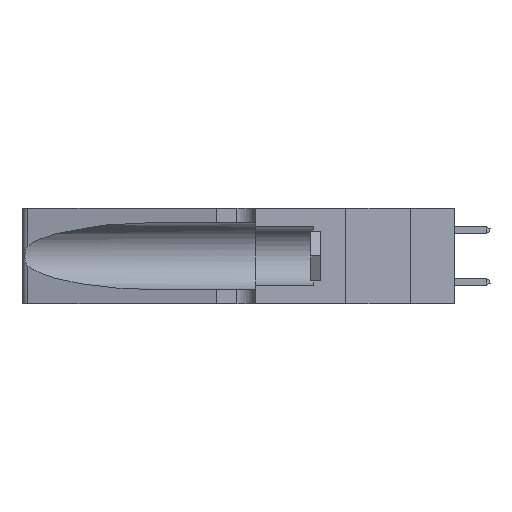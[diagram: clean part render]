
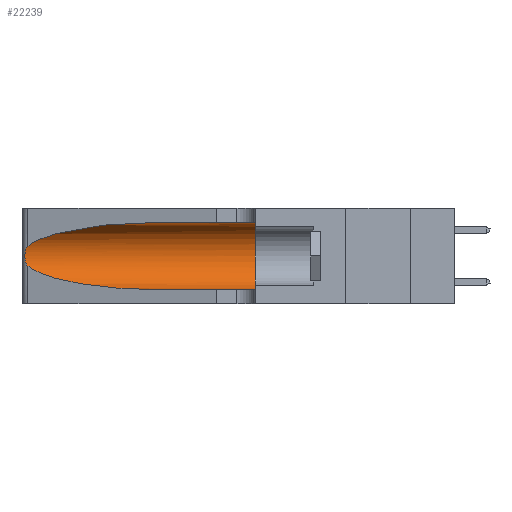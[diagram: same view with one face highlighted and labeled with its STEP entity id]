
A CAD part, left-side view. The second image highlights one B-rep face of the part: STEP entity #22239.
In plain terms, the highlighted cylindrical face has radius 3.308 mm (diameter 6.617 mm), a partial arc.
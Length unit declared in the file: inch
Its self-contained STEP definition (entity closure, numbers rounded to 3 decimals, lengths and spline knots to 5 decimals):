
#1173 = VERTEX_POINT ( 'NONE', #2139 ) ;
#2036 = LINE ( 'NONE', #36494, #19324 ) ;
#2139 = CARTESIAN_POINT ( 'NONE',  ( 0.1305, 0.35, 0.05475 ) ) ;
#3150 = CARTESIAN_POINT ( 'NONE',  ( 0.26018, 1.23835, 0.19895 ) ) ;
#3463 = CARTESIAN_POINT ( 'NONE',  ( 0.18966, 0.96281, 0.05475 ) ) ;
#4103 = EDGE_CURVE ( 'NONE', #9944, #24727, #31185, .T. ) ;
#5092 = VECTOR ( 'NONE', #9579, 39.37008 ) ;
#6643 = CARTESIAN_POINT ( 'NONE',  ( 0.26075, 1.23896, 0.178 ) ) ;
#7323 = CYLINDRICAL_SURFACE ( 'NONE', #28045, 0.13025 ) ;
#8368 = VERTEX_POINT ( 'NONE', #39173 ) ;
#8820 = CARTESIAN_POINT ( 'NONE',  ( 0.1305, 0.35, 0.185 ) ) ;
#8962 = VERTEX_POINT ( 'NONE', #18422 ) ;
#9579 = DIRECTION ( 'NONE',  ( 0., -1., 0. ) ) ;
#9944 = VERTEX_POINT ( 'NONE', #30149 ) ;
#9974 = CARTESIAN_POINT ( 'NONE',  ( 0.18966, 0.96281, 0.31525 ) ) ;
#10121 = CARTESIAN_POINT ( 'NONE',  ( 0.25856, 1.23593, 0.16098 ) ) ;
#10421 = CARTESIAN_POINT ( 'NONE',  ( 0.25487, 1.22718, 0.14631 ) ) ;
#12302 = DIRECTION ( 'NONE',  ( 0., 0., 1. ) ) ;
#13453 = CARTESIAN_POINT ( 'NONE',  ( 0.25487, 1.22718, 0.22369 ) ) ;
#13593 = CARTESIAN_POINT ( 'NONE',  ( 0.25639, 1.23186, 0.15144 ) ) ;
#15755 = CARTESIAN_POINT ( 'NONE',  ( 0.1305, 0.72297, 0.05475 ) ) ;
#16517 = EDGE_CURVE ( 'NONE', #8368, #8962, #23408, .T. ) ;
#17034 = CARTESIAN_POINT ( 'NONE',  ( 0.25487, 1.22718, 0.14631 ) ) ;
#18422 = CARTESIAN_POINT ( 'NONE',  ( 0.1305, 0.35, 0.31525 ) ) ;
#19324 = VECTOR ( 'NONE', #39889, 39.37008 ) ;
#19379 = ORIENTED_EDGE ( 'NONE', *, *, #30400, .F. ) ;
#20198 = CARTESIAN_POINT ( 'NONE',  ( 0.25555, 1.22994, 0.2215 ) ) ;
#20310 = CIRCLE ( 'NONE', #35894, 0.13025 ) ;
#20346 = CARTESIAN_POINT ( 'NONE',  ( 0.25639, 1.23184, 0.21858 ) ) ;
#20348 = CARTESIAN_POINT ( 'NONE',  ( 0.25487, 1.22718, 0.22369 ) ) ;
#22239 = ADVANCED_FACE ( 'NONE', ( #34654 ), #7323, .F. ) ;
#22637 = ORIENTED_EDGE ( 'NONE', *, *, #16517, .F. ) ;
#23408 = LINE ( 'NONE', #36947, #5092 ) ;
#23769 = CARTESIAN_POINT ( 'NONE',  ( 0.25854, 1.2359, 0.20912 ) ) ;
#24727 = VERTEX_POINT ( 'NONE', #15755 ) ;
#25240 = ORIENTED_EDGE ( 'NONE', *, *, #44294, .T. ) ;
#27221 = CARTESIAN_POINT ( 'NONE',  ( 0.26075, 1.23896, 0.19203 ) ) ;
#27389 = VERTEX_POINT ( 'NONE', #29786 ) ;
#27517 = EDGE_CURVE ( 'NONE', #27389, #9944, #27940, .T. ) ;
#27535 = CARTESIAN_POINT ( 'NONE',  ( 0.2373, 1.15595, 0.08982 ) ) ;
#27940 = B_SPLINE_CURVE_WITH_KNOTS ( 'NONE', 3,
 ( #13453, #20198, #20346, #44138, #23769, #3150, #27221, #6643, #30638, #10121, #34060, #13593, #37480, #17034 ),
 .UNSPECIFIED., .F., .F.,
 ( 4, 2, 2, 2, 2, 2, 4 ),
 ( 0., 0.00027, 0.00053, 0.00107, 0.0016, 0.00187, 0.00214 ),
 .UNSPECIFIED. ) ;
#28045 = AXIS2_PLACEMENT_3D ( 'NONE', #33790, #37069, #30377 ) ;
#29151 = EDGE_LOOP ( 'NONE', ( #25240, #32268, #29885, #43874, #19379, #22637 ) ) ;
#29786 = CARTESIAN_POINT ( 'NONE',  ( 0.25487, 1.22718, 0.22369 ) ) ;
#29885 = ORIENTED_EDGE ( 'NONE', *, *, #4103, .T. ) ;
#30149 = CARTESIAN_POINT ( 'NONE',  ( 0.25487, 1.22718, 0.14631 ) ) ;
#30377 = DIRECTION ( 'NONE',  ( 0., 0., -1. ) ) ;
#30400 = EDGE_CURVE ( 'NONE', #8962, #1173, #20310, .T. ) ;
#30638 = CARTESIAN_POINT ( 'NONE',  ( 0.26017, 1.23833, 0.17102 ) ) ;
#31185 =( BOUNDED_CURVE ( )  B_SPLINE_CURVE ( 3, ( #10421, #27535, #3463, #34355 ),
 .UNSPECIFIED., .F., .T. ) 
 B_SPLINE_CURVE_WITH_KNOTS ( ( 4, 4 ),
 ( 3.44316, 4.71239 ),
 .UNSPECIFIED. ) 
 CURVE ( )  GEOMETRIC_REPRESENTATION_ITEM ( )  RATIONAL_B_SPLINE_CURVE ( ( 1., 0.87, 0.87, 1. ) ) 
 REPRESENTATION_ITEM ( '' )  );
#32268 = ORIENTED_EDGE ( 'NONE', *, *, #27517, .T. ) ;
#32555 =( BOUNDED_CURVE ( )  B_SPLINE_CURVE ( 3, ( #37341, #9974, #40719, #20348 ),
 .UNSPECIFIED., .F., .F. ) 
 B_SPLINE_CURVE_WITH_KNOTS ( ( 4, 4 ),
 ( 1.5708, 2.84003 ),
 .UNSPECIFIED. ) 
 CURVE ( )  GEOMETRIC_REPRESENTATION_ITEM ( )  RATIONAL_B_SPLINE_CURVE ( ( 1., 0.87, 0.87, 1. ) ) 
 REPRESENTATION_ITEM ( '' )  );
#32786 = DIRECTION ( 'NONE',  ( 0., 1., 0. ) ) ;
#33790 = CARTESIAN_POINT ( 'NONE',  ( 0.1305, 1.61858, 0.185 ) ) ;
#34060 = CARTESIAN_POINT ( 'NONE',  ( 0.25789, 1.23486, 0.15765 ) ) ;
#34160 = EDGE_CURVE ( 'NONE', #24727, #1173, #2036, .T. ) ;
#34355 = CARTESIAN_POINT ( 'NONE',  ( 0.1305, 0.72297, 0.05475 ) ) ;
#34654 = FACE_OUTER_BOUND ( 'NONE', #29151, .T. ) ;
#35894 = AXIS2_PLACEMENT_3D ( 'NONE', #8820, #32786, #12302 ) ;
#36494 = CARTESIAN_POINT ( 'NONE',  ( 0.1305, 1.61858, 0.05475 ) ) ;
#36947 = CARTESIAN_POINT ( 'NONE',  ( 0.1305, 1.61858, 0.31525 ) ) ;
#37069 = DIRECTION ( 'NONE',  ( 0., -1., 0. ) ) ;
#37341 = CARTESIAN_POINT ( 'NONE',  ( 0.1305, 0.72297, 0.31525 ) ) ;
#37480 = CARTESIAN_POINT ( 'NONE',  ( 0.25555, 1.22993, 0.14849 ) ) ;
#39173 = CARTESIAN_POINT ( 'NONE',  ( 0.1305, 0.72297, 0.31525 ) ) ;
#39889 = DIRECTION ( 'NONE',  ( 0., -1., 0. ) ) ;
#40719 = CARTESIAN_POINT ( 'NONE',  ( 0.2373, 1.15595, 0.28018 ) ) ;
#43874 = ORIENTED_EDGE ( 'NONE', *, *, #34160, .T. ) ;
#44138 = CARTESIAN_POINT ( 'NONE',  ( 0.25787, 1.23484, 0.2124 ) ) ;
#44294 = EDGE_CURVE ( 'NONE', #8368, #27389, #32555, .T. ) ;
